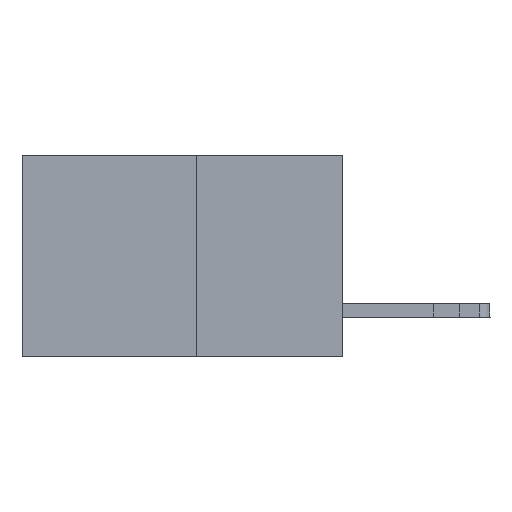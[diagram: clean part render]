
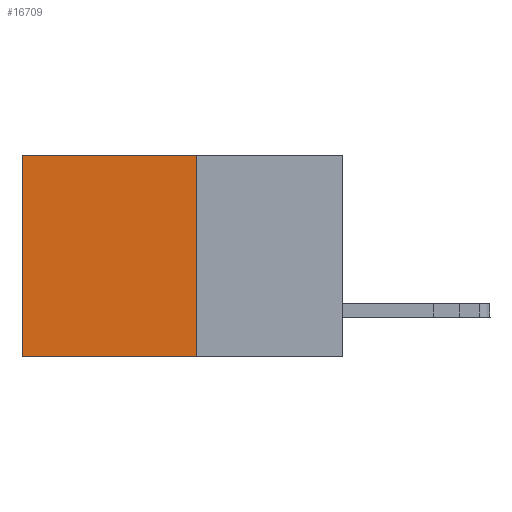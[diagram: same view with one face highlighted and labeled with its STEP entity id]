
A CAD part, left-side view. The second image highlights one B-rep face of the part: STEP entity #16709.
In plain terms, the highlighted planar face has unit normal (-1, 0, 0).
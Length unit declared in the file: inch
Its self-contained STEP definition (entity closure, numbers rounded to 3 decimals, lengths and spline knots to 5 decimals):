
#49 = EDGE_CURVE ( 'NONE', #6255, #14760, #13414, .T. ) ;
#228 = VECTOR ( 'NONE', #2200, 39.37008 ) ;
#536 = CARTESIAN_POINT ( 'NONE',  ( 0.277, 0.59, 0. ) ) ;
#1705 = CARTESIAN_POINT ( 'NONE',  ( 0.277, 0.27, -0.37 ) ) ;
#2200 = DIRECTION ( 'NONE',  ( 0., 0., -1. ) ) ;
#2560 = DIRECTION ( 'NONE',  ( 0., 0., -1. ) ) ;
#2739 = AXIS2_PLACEMENT_3D ( 'NONE', #10595, #9136, #2560 ) ;
#2820 = EDGE_LOOP ( 'NONE', ( #7791, #12819, #3744, #17403 ) ) ;
#3547 = DIRECTION ( 'NONE',  ( 0., 1., 0. ) ) ;
#3744 = ORIENTED_EDGE ( 'NONE', *, *, #10115, .F. ) ;
#4596 = VERTEX_POINT ( 'NONE', #536 ) ;
#4674 = CARTESIAN_POINT ( 'NONE',  ( 0.277, 0.27, 0. ) ) ;
#4724 = LINE ( 'NONE', #10303, #11859 ) ;
#6255 = VERTEX_POINT ( 'NONE', #1705 ) ;
#7791 = ORIENTED_EDGE ( 'NONE', *, *, #9154, .T. ) ;
#9136 = DIRECTION ( 'NONE',  ( 1., 0., 0. ) ) ;
#9154 = EDGE_CURVE ( 'NONE', #4596, #14760, #4724, .T. ) ;
#9319 = FACE_OUTER_BOUND ( 'NONE', #2820, .T. ) ;
#10115 = EDGE_CURVE ( 'NONE', #16808, #6255, #14957, .T. ) ;
#10303 = CARTESIAN_POINT ( 'NONE',  ( 0.277, 0.59, -0.37 ) ) ;
#10517 = CARTESIAN_POINT ( 'NONE',  ( 0.277, 0.27, -0.37 ) ) ;
#10595 = CARTESIAN_POINT ( 'NONE',  ( 0.277, 0.27, -0.37 ) ) ;
#10940 = DIRECTION ( 'NONE',  ( 0., 1., 0. ) ) ;
#11071 = VECTOR ( 'NONE', #3547, 39.37008 ) ;
#11859 = VECTOR ( 'NONE', #12760, 39.37008 ) ;
#12345 = VECTOR ( 'NONE', #10940, 39.37008 ) ;
#12435 = EDGE_CURVE ( 'NONE', #16808, #4596, #13498, .T. ) ;
#12760 = DIRECTION ( 'NONE',  ( 0., 0., -1. ) ) ;
#12819 = ORIENTED_EDGE ( 'NONE', *, *, #49, .F. ) ;
#13414 = LINE ( 'NONE', #13763, #12345 ) ;
#13498 = LINE ( 'NONE', #14858, #11071 ) ;
#13510 = PLANE ( 'NONE',  #2739 ) ;
#13763 = CARTESIAN_POINT ( 'NONE',  ( 0.277, 0.27, -0.37 ) ) ;
#14760 = VERTEX_POINT ( 'NONE', #14945 ) ;
#14858 = CARTESIAN_POINT ( 'NONE',  ( 0.277, 0.27, 0. ) ) ;
#14945 = CARTESIAN_POINT ( 'NONE',  ( 0.277, 0.59, -0.37 ) ) ;
#14957 = LINE ( 'NONE', #10517, #228 ) ;
#16709 = ADVANCED_FACE ( 'NONE', ( #9319 ), #13510, .F. ) ;
#16808 = VERTEX_POINT ( 'NONE', #4674 ) ;
#17403 = ORIENTED_EDGE ( 'NONE', *, *, #12435, .T. ) ;
